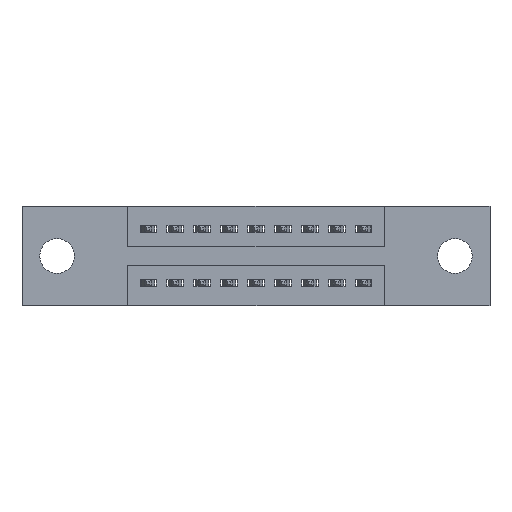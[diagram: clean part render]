
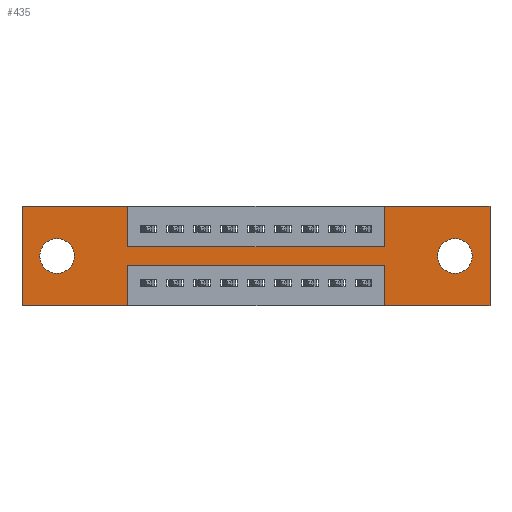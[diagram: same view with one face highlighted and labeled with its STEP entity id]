
A CAD part, front view. The second image highlights one B-rep face of the part: STEP entity #435.
In plain terms, the highlighted planar face has unit normal (0, -1, 0).
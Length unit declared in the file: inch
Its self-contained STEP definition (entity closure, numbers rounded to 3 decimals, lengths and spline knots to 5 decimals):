
#54 = DIRECTION ( 'NONE',  ( 0., 0., -1. ) ) ;
#67 = ORIENTED_EDGE ( 'NONE', *, *, #687, .F. ) ;
#227 = VECTOR ( 'NONE', #7339, 39.37008 ) ;
#291 = EDGE_CURVE ( 'NONE', #9508, #3691, #10330, .T. ) ;
#360 = CARTESIAN_POINT ( 'NONE',  ( 0., 0., 0. ) ) ;
#435 = ADVANCED_FACE ( 'NONE', ( #1967, #5863, #4884 ), #11521, .T. ) ;
#493 = AXIS2_PLACEMENT_3D ( 'NONE', #4547, #6398, #3752 ) ;
#537 = CARTESIAN_POINT ( 'NONE',  ( 0.3925, 0., -0.15 ) ) ;
#548 = AXIS2_PLACEMENT_3D ( 'NONE', #11439, #6100, #766 ) ;
#687 = EDGE_CURVE ( 'NONE', #5245, #9870, #4773, .T. ) ;
#766 = DIRECTION ( 'NONE',  ( 0., 0., -1. ) ) ;
#808 = ORIENTED_EDGE ( 'NONE', *, *, #10765, .T. ) ;
#861 = DIRECTION ( 'NONE',  ( 0., -1., 0. ) ) ;
#884 = CARTESIAN_POINT ( 'NONE',  ( 0., 0., 0. ) ) ;
#956 = VERTEX_POINT ( 'NONE', #8755 ) ;
#1021 = AXIS2_PLACEMENT_3D ( 'NONE', #7951, #6189, #2721 ) ;
#1116 = CARTESIAN_POINT ( 'NONE',  ( 0., 0., -0.37 ) ) ;
#1144 = DIRECTION ( 'NONE',  ( 0., 0., -1. ) ) ;
#1183 = VECTOR ( 'NONE', #3810, 39.37008 ) ;
#1233 = CARTESIAN_POINT ( 'NONE',  ( 0.13, 0., -0.185 ) ) ;
#1428 = ORIENTED_EDGE ( 'NONE', *, *, #3617, .F. ) ;
#1514 = EDGE_CURVE ( 'NONE', #10415, #6311, #5840, .T. ) ;
#1637 = VECTOR ( 'NONE', #2732, 39.37008 ) ;
#1648 = VERTEX_POINT ( 'NONE', #2031 ) ;
#1752 = EDGE_CURVE ( 'NONE', #9144, #956, #2892, .T. ) ;
#1895 = LINE ( 'NONE', #1116, #1637 ) ;
#1967 = FACE_BOUND ( 'NONE', #5816, .T. ) ;
#2031 = CARTESIAN_POINT ( 'NONE',  ( 1.735, 0., 0. ) ) ;
#2128 = DIRECTION ( 'NONE',  ( 0., 1., 0. ) ) ;
#2205 = VECTOR ( 'NONE', #4862, 39.37008 ) ;
#2310 = LINE ( 'NONE', #7213, #227 ) ;
#2444 = CARTESIAN_POINT ( 'NONE',  ( 0.13, 0., -0.121 ) ) ;
#2462 = CARTESIAN_POINT ( 'NONE',  ( 1.605, 0., -0.249 ) ) ;
#2523 = VECTOR ( 'NONE', #4187, 39.37008 ) ;
#2719 = CARTESIAN_POINT ( 'NONE',  ( 1.3425, 0., 0. ) ) ;
#2721 = DIRECTION ( 'NONE',  ( 0., 0., -1. ) ) ;
#2732 = DIRECTION ( 'NONE',  ( -1., 0., 0. ) ) ;
#2821 = DIRECTION ( 'NONE',  ( 0., 0., 1. ) ) ;
#2892 = LINE ( 'NONE', #8280, #2205 ) ;
#2943 = CARTESIAN_POINT ( 'NONE',  ( 0.3925, 0., -0.37 ) ) ;
#3028 = ORIENTED_EDGE ( 'NONE', *, *, #11532, .F. ) ;
#3306 = VECTOR ( 'NONE', #11185, 39.37008 ) ;
#3308 = ORIENTED_EDGE ( 'NONE', *, *, #8768, .T. ) ;
#3394 = LINE ( 'NONE', #5725, #1183 ) ;
#3402 = DIRECTION ( 'NONE',  ( 0., 0., 1. ) ) ;
#3409 = LINE ( 'NONE', #7746, #6617 ) ;
#3617 = EDGE_CURVE ( 'NONE', #956, #5449, #2310, .T. ) ;
#3638 = VERTEX_POINT ( 'NONE', #2719 ) ;
#3691 = VERTEX_POINT ( 'NONE', #9132 ) ;
#3752 = DIRECTION ( 'NONE',  ( 0., 0., 1. ) ) ;
#3810 = DIRECTION ( 'NONE',  ( -1., 0., 0. ) ) ;
#3913 = EDGE_CURVE ( 'NONE', #5255, #9144, #3409, .T. ) ;
#4049 = EDGE_CURVE ( 'NONE', #4572, #5255, #1895, .T. ) ;
#4108 = CARTESIAN_POINT ( 'NONE',  ( 0., 0., 0. ) ) ;
#4187 = DIRECTION ( 'NONE',  ( 0., 0., 1. ) ) ;
#4534 = CIRCLE ( 'NONE', #493, 0.064 ) ;
#4547 = CARTESIAN_POINT ( 'NONE',  ( 0.13, 0., -0.185 ) ) ;
#4572 = VERTEX_POINT ( 'NONE', #9668 ) ;
#4773 = LINE ( 'NONE', #10037, #5010 ) ;
#4862 = DIRECTION ( 'NONE',  ( -1., 0., 0. ) ) ;
#4884 = FACE_OUTER_BOUND ( 'NONE', #10311, .T. ) ;
#4897 = VECTOR ( 'NONE', #54, 39.37008 ) ;
#4954 = EDGE_CURVE ( 'NONE', #5449, #9508, #3394, .T. ) ;
#4989 = CARTESIAN_POINT ( 'NONE',  ( 1.3425, 0., -0.22 ) ) ;
#5010 = VECTOR ( 'NONE', #1144, 39.37008 ) ;
#5177 = CARTESIAN_POINT ( 'NONE',  ( 1.3425, 0., -0.37 ) ) ;
#5245 = VERTEX_POINT ( 'NONE', #8670 ) ;
#5255 = VERTEX_POINT ( 'NONE', #5177 ) ;
#5374 = EDGE_CURVE ( 'NONE', #6311, #10415, #7820, .T. ) ;
#5393 = DIRECTION ( 'NONE',  ( 1., 0., 0. ) ) ;
#5433 = VERTEX_POINT ( 'NONE', #9987 ) ;
#5449 = VERTEX_POINT ( 'NONE', #2943 ) ;
#5725 = CARTESIAN_POINT ( 'NONE',  ( 0., 0., -0.37 ) ) ;
#5816 = EDGE_LOOP ( 'NONE', ( #10919, #6891 ) ) ;
#5840 = CIRCLE ( 'NONE', #1021, 0.064 ) ;
#5863 = FACE_BOUND ( 'NONE', #7527, .T. ) ;
#5906 = ORIENTED_EDGE ( 'NONE', *, *, #10644, .F. ) ;
#5999 = EDGE_CURVE ( 'NONE', #3638, #1648, #11289, .T. ) ;
#6100 = DIRECTION ( 'NONE',  ( 0., 1., 0. ) ) ;
#6189 = DIRECTION ( 'NONE',  ( 0., 1., 0. ) ) ;
#6311 = VERTEX_POINT ( 'NONE', #10897 ) ;
#6398 = DIRECTION ( 'NONE',  ( 0., 1., 0. ) ) ;
#6413 = VECTOR ( 'NONE', #10364, 39.37008 ) ;
#6568 = LINE ( 'NONE', #10650, #4897 ) ;
#6617 = VECTOR ( 'NONE', #3402, 39.37008 ) ;
#6891 = ORIENTED_EDGE ( 'NONE', *, *, #1514, .T. ) ;
#6965 = CARTESIAN_POINT ( 'NONE',  ( 0., 0., -0.37 ) ) ;
#7064 = DIRECTION ( 'NONE',  ( 0., 0., -1. ) ) ;
#7209 = ORIENTED_EDGE ( 'NONE', *, *, #4954, .F. ) ;
#7213 = CARTESIAN_POINT ( 'NONE',  ( 0.3925, 0., -0.37 ) ) ;
#7221 = ORIENTED_EDGE ( 'NONE', *, *, #1752, .F. ) ;
#7249 = AXIS2_PLACEMENT_3D ( 'NONE', #6965, #861, #7064 ) ;
#7331 = ORIENTED_EDGE ( 'NONE', *, *, #10064, .F. ) ;
#7339 = DIRECTION ( 'NONE',  ( 0., 0., -1. ) ) ;
#7373 = ORIENTED_EDGE ( 'NONE', *, *, #4049, .F. ) ;
#7527 = EDGE_LOOP ( 'NONE', ( #808, #3308 ) ) ;
#7560 = ORIENTED_EDGE ( 'NONE', *, *, #291, .F. ) ;
#7659 = ORIENTED_EDGE ( 'NONE', *, *, #5999, .F. ) ;
#7746 = CARTESIAN_POINT ( 'NONE',  ( 1.3425, 0., -0.37 ) ) ;
#7750 = DIRECTION ( 'NONE',  ( 1., 0., 0. ) ) ;
#7820 = CIRCLE ( 'NONE', #548, 0.064 ) ;
#7891 = EDGE_CURVE ( 'NONE', #3691, #5245, #7999, .T. ) ;
#7951 = CARTESIAN_POINT ( 'NONE',  ( 1.605, 0., -0.185 ) ) ;
#7999 = LINE ( 'NONE', #360, #3306 ) ;
#8014 = AXIS2_PLACEMENT_3D ( 'NONE', #1233, #2128, #2821 ) ;
#8280 = CARTESIAN_POINT ( 'NONE',  ( 0.3925, 0., -0.22 ) ) ;
#8333 = CARTESIAN_POINT ( 'NONE',  ( 0.13, 0., -0.249 ) ) ;
#8532 = LINE ( 'NONE', #537, #11189 ) ;
#8600 = VERTEX_POINT ( 'NONE', #2444 ) ;
#8670 = CARTESIAN_POINT ( 'NONE',  ( 0.3925, 0., 0. ) ) ;
#8755 = CARTESIAN_POINT ( 'NONE',  ( 0.3925, 0., -0.22 ) ) ;
#8768 = EDGE_CURVE ( 'NONE', #11364, #8600, #4534, .T. ) ;
#8915 = VECTOR ( 'NONE', #5393, 39.37008 ) ;
#9132 = CARTESIAN_POINT ( 'NONE',  ( 0., 0., 0. ) ) ;
#9144 = VERTEX_POINT ( 'NONE', #4989 ) ;
#9508 = VERTEX_POINT ( 'NONE', #10012 ) ;
#9512 = CARTESIAN_POINT ( 'NONE',  ( 0.3925, 0., -0.15 ) ) ;
#9668 = CARTESIAN_POINT ( 'NONE',  ( 1.735, 0., -0.37 ) ) ;
#9870 = VERTEX_POINT ( 'NONE', #9512 ) ;
#9987 = CARTESIAN_POINT ( 'NONE',  ( 1.3425, 0., -0.15 ) ) ;
#10012 = CARTESIAN_POINT ( 'NONE',  ( 0., 0., -0.37 ) ) ;
#10037 = CARTESIAN_POINT ( 'NONE',  ( 0.3925, 0., 0. ) ) ;
#10064 = EDGE_CURVE ( 'NONE', #9870, #5433, #8532, .T. ) ;
#10188 = CIRCLE ( 'NONE', #8014, 0.064 ) ;
#10311 = EDGE_LOOP ( 'NONE', ( #1428, #7221, #10996, #7373, #5906, #7659, #3028, #7331, #67, #11104, #7560, #7209 ) ) ;
#10330 = LINE ( 'NONE', #4108, #6413 ) ;
#10364 = DIRECTION ( 'NONE',  ( 0., 0., 1. ) ) ;
#10415 = VERTEX_POINT ( 'NONE', #2462 ) ;
#10644 = EDGE_CURVE ( 'NONE', #1648, #4572, #6568, .T. ) ;
#10650 = CARTESIAN_POINT ( 'NONE',  ( 1.735, 0., 0. ) ) ;
#10765 = EDGE_CURVE ( 'NONE', #8600, #11364, #10188, .T. ) ;
#10897 = CARTESIAN_POINT ( 'NONE',  ( 1.605, 0., -0.121 ) ) ;
#10919 = ORIENTED_EDGE ( 'NONE', *, *, #5374, .T. ) ;
#10996 = ORIENTED_EDGE ( 'NONE', *, *, #3913, .F. ) ;
#11104 = ORIENTED_EDGE ( 'NONE', *, *, #7891, .F. ) ;
#11185 = DIRECTION ( 'NONE',  ( 1., 0., 0. ) ) ;
#11189 = VECTOR ( 'NONE', #7750, 39.37008 ) ;
#11289 = LINE ( 'NONE', #884, #8915 ) ;
#11300 = LINE ( 'NONE', #11382, #2523 ) ;
#11364 = VERTEX_POINT ( 'NONE', #8333 ) ;
#11382 = CARTESIAN_POINT ( 'NONE',  ( 1.3425, 0., 0. ) ) ;
#11439 = CARTESIAN_POINT ( 'NONE',  ( 1.605, 0., -0.185 ) ) ;
#11521 = PLANE ( 'NONE',  #7249 ) ;
#11532 = EDGE_CURVE ( 'NONE', #5433, #3638, #11300, .T. ) ;
